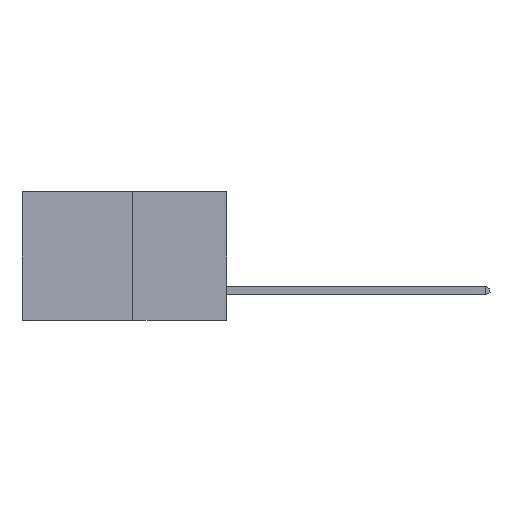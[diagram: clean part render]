
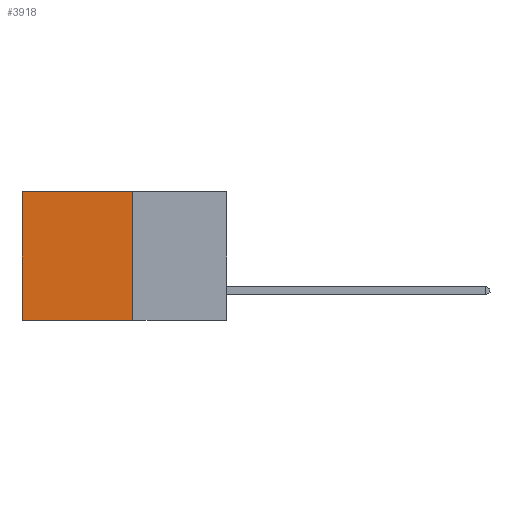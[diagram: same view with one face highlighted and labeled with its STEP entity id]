
A CAD part, left-side view. The second image highlights one B-rep face of the part: STEP entity #3918.
In plain terms, the highlighted planar face has unit normal (-1, 0, 0).
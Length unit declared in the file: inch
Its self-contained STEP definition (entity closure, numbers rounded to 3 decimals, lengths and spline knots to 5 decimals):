
#997 = FACE_OUTER_BOUND ( 'NONE', #1669, .T. ) ;
#1337 = CARTESIAN_POINT ( 'NONE',  ( 0.277, 0.59, -0.37 ) ) ;
#1422 = DIRECTION ( 'NONE',  ( 0., 1., 0. ) ) ;
#1669 = EDGE_LOOP ( 'NONE', ( #2148, #2031, #2085, #1959 ) ) ;
#1785 = LINE ( 'NONE', #1337, #2107 ) ;
#1959 = ORIENTED_EDGE ( 'NONE', *, *, #5973, .T. ) ;
#2031 = ORIENTED_EDGE ( 'NONE', *, *, #10965, .F. ) ;
#2085 = ORIENTED_EDGE ( 'NONE', *, *, #6660, .F. ) ;
#2107 = VECTOR ( 'NONE', #7435, 39.37008 ) ;
#2148 = ORIENTED_EDGE ( 'NONE', *, *, #6981, .T. ) ;
#2558 = LINE ( 'NONE', #9597, #5313 ) ;
#3530 = VERTEX_POINT ( 'NONE', #8246 ) ;
#3918 = ADVANCED_FACE ( 'NONE', ( #997 ), #10644, .F. ) ;
#4220 = CARTESIAN_POINT ( 'NONE',  ( 0.277, 0.59, -0.37 ) ) ;
#4475 = DIRECTION ( 'NONE',  ( 1., 0., 0. ) ) ;
#4843 = VERTEX_POINT ( 'NONE', #4220 ) ;
#4914 = CARTESIAN_POINT ( 'NONE',  ( 0.277, 0.27, -0.37 ) ) ;
#5313 = VECTOR ( 'NONE', #9390, 39.37008 ) ;
#5659 = CARTESIAN_POINT ( 'NONE',  ( 0.277, 0.59, 0. ) ) ;
#5973 = EDGE_CURVE ( 'NONE', #3530, #6274, #2558, .T. ) ;
#6274 = VERTEX_POINT ( 'NONE', #5659 ) ;
#6660 = EDGE_CURVE ( 'NONE', #3530, #9931, #8834, .T. ) ;
#6981 = EDGE_CURVE ( 'NONE', #6274, #4843, #1785, .T. ) ;
#7435 = DIRECTION ( 'NONE',  ( 0., 0., -1. ) ) ;
#7887 = LINE ( 'NONE', #10616, #8135 ) ;
#8135 = VECTOR ( 'NONE', #1422, 39.37008 ) ;
#8246 = CARTESIAN_POINT ( 'NONE',  ( 0.277, 0.27, 0. ) ) ;
#8834 = LINE ( 'NONE', #4914, #10877 ) ;
#9390 = DIRECTION ( 'NONE',  ( 0., 1., 0. ) ) ;
#9597 = CARTESIAN_POINT ( 'NONE',  ( 0.277, 0.27, 0. ) ) ;
#9613 = CARTESIAN_POINT ( 'NONE',  ( 0.277, 0.27, -0.37 ) ) ;
#9931 = VERTEX_POINT ( 'NONE', #9613 ) ;
#10272 = CARTESIAN_POINT ( 'NONE',  ( 0.277, 0.27, -0.37 ) ) ;
#10296 = DIRECTION ( 'NONE',  ( 0., 0., -1. ) ) ;
#10554 = DIRECTION ( 'NONE',  ( 0., 0., -1. ) ) ;
#10616 = CARTESIAN_POINT ( 'NONE',  ( 0.277, 0.27, -0.37 ) ) ;
#10634 = AXIS2_PLACEMENT_3D ( 'NONE', #10272, #4475, #10296 ) ;
#10644 = PLANE ( 'NONE',  #10634 ) ;
#10877 = VECTOR ( 'NONE', #10554, 39.37008 ) ;
#10965 = EDGE_CURVE ( 'NONE', #9931, #4843, #7887, .T. ) ;
